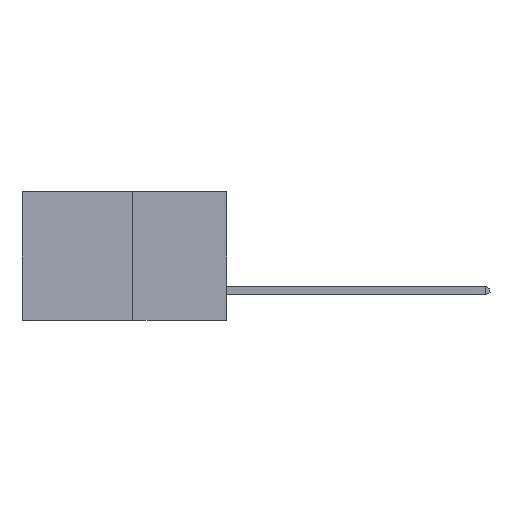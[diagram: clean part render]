
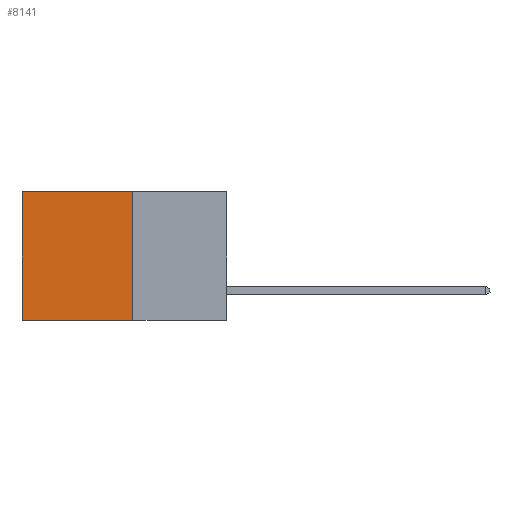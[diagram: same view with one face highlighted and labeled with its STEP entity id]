
A CAD part, left-side view. The second image highlights one B-rep face of the part: STEP entity #8141.
In plain terms, the highlighted planar face has unit normal (-1, 0, 0).
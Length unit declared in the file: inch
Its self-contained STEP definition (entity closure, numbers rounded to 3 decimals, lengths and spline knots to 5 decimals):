
#309 = CARTESIAN_POINT ( 'NONE',  ( 0.277, 0.27, -0.37 ) ) ;
#1213 = LINE ( 'NONE', #5488, #10804 ) ;
#1271 = DIRECTION ( 'NONE',  ( 0., 0., -1. ) ) ;
#1805 = VECTOR ( 'NONE', #10398, 39.37008 ) ;
#1936 = EDGE_LOOP ( 'NONE', ( #8836, #10860, #3156, #2893 ) ) ;
#2870 = VERTEX_POINT ( 'NONE', #10975 ) ;
#2893 = ORIENTED_EDGE ( 'NONE', *, *, #9933, .T. ) ;
#2932 = DIRECTION ( 'NONE',  ( 0., 1., 0. ) ) ;
#2999 = EDGE_CURVE ( 'NONE', #6594, #2870, #1213, .T. ) ;
#3008 = CARTESIAN_POINT ( 'NONE',  ( 0.277, 0.27, 0. ) ) ;
#3156 = ORIENTED_EDGE ( 'NONE', *, *, #6138, .F. ) ;
#3436 = AXIS2_PLACEMENT_3D ( 'NONE', #309, #6791, #1271 ) ;
#3509 = VECTOR ( 'NONE', #5891, 39.37008 ) ;
#3705 = LINE ( 'NONE', #8274, #5859 ) ;
#3802 = LINE ( 'NONE', #7730, #3509 ) ;
#4162 = EDGE_CURVE ( 'NONE', #4987, #2870, #3705, .T. ) ;
#4206 = CARTESIAN_POINT ( 'NONE',  ( 0.277, 0.27, 0. ) ) ;
#4274 = LINE ( 'NONE', #4206, #1805 ) ;
#4974 = PLANE ( 'NONE',  #3436 ) ;
#4987 = VERTEX_POINT ( 'NONE', #8228 ) ;
#5488 = CARTESIAN_POINT ( 'NONE',  ( 0.277, 0.27, -0.37 ) ) ;
#5859 = VECTOR ( 'NONE', #7969, 39.37008 ) ;
#5891 = DIRECTION ( 'NONE',  ( 0., 0., -1. ) ) ;
#6138 = EDGE_CURVE ( 'NONE', #6342, #6594, #3802, .T. ) ;
#6342 = VERTEX_POINT ( 'NONE', #3008 ) ;
#6594 = VERTEX_POINT ( 'NONE', #7391 ) ;
#6791 = DIRECTION ( 'NONE',  ( 1., 0., 0. ) ) ;
#7391 = CARTESIAN_POINT ( 'NONE',  ( 0.277, 0.27, -0.37 ) ) ;
#7730 = CARTESIAN_POINT ( 'NONE',  ( 0.277, 0.27, -0.37 ) ) ;
#7969 = DIRECTION ( 'NONE',  ( 0., 0., -1. ) ) ;
#8141 = ADVANCED_FACE ( 'NONE', ( #9503 ), #4974, .F. ) ;
#8228 = CARTESIAN_POINT ( 'NONE',  ( 0.277, 0.59, 0. ) ) ;
#8274 = CARTESIAN_POINT ( 'NONE',  ( 0.277, 0.59, -0.37 ) ) ;
#8836 = ORIENTED_EDGE ( 'NONE', *, *, #4162, .T. ) ;
#9503 = FACE_OUTER_BOUND ( 'NONE', #1936, .T. ) ;
#9933 = EDGE_CURVE ( 'NONE', #6342, #4987, #4274, .T. ) ;
#10398 = DIRECTION ( 'NONE',  ( 0., 1., 0. ) ) ;
#10804 = VECTOR ( 'NONE', #2932, 39.37008 ) ;
#10860 = ORIENTED_EDGE ( 'NONE', *, *, #2999, .F. ) ;
#10975 = CARTESIAN_POINT ( 'NONE',  ( 0.277, 0.59, -0.37 ) ) ;
